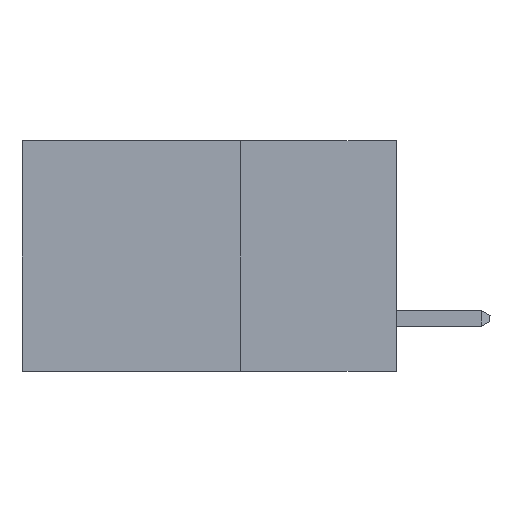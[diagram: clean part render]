
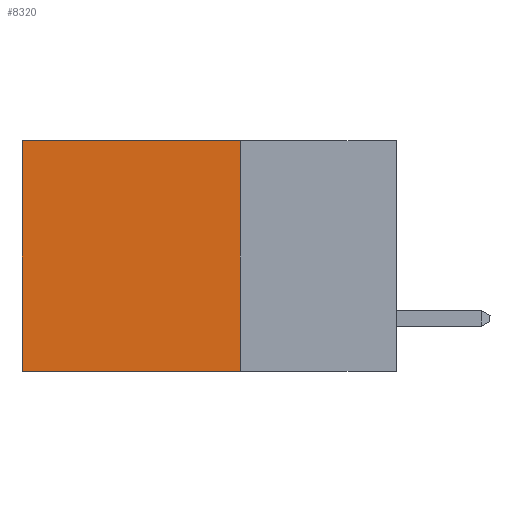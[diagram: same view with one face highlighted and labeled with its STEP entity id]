
A CAD part, left-side view. The second image highlights one B-rep face of the part: STEP entity #8320.
In plain terms, the highlighted planar face has unit normal (-1, 0, 0).
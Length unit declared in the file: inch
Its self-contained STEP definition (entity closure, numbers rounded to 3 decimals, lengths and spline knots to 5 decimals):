
#2865 = ORIENTED_EDGE ( 'NONE', *, *, #7196, .T. ) ;
#3158 = CARTESIAN_POINT ( 'NONE',  ( 0.2615, 0.25, -0.37 ) ) ;
#3187 = VERTEX_POINT ( 'NONE', #3698 ) ;
#3439 = EDGE_CURVE ( 'NONE', #10268, #3187, #15958, .T. ) ;
#3698 = CARTESIAN_POINT ( 'NONE',  ( 0.2615, 0.6, 0. ) ) ;
#4251 = VERTEX_POINT ( 'NONE', #8375 ) ;
#4569 = FACE_OUTER_BOUND ( 'NONE', #12228, .T. ) ;
#5017 = EDGE_CURVE ( 'NONE', #10268, #4251, #17143, .T. ) ;
#7196 = EDGE_CURVE ( 'NONE', #3187, #14662, #18807, .T. ) ;
#7210 = CARTESIAN_POINT ( 'NONE',  ( 0.2615, 0.6, -0.37 ) ) ;
#8123 = CARTESIAN_POINT ( 'NONE',  ( 0.2615, 0.6, -0.37 ) ) ;
#8320 = ADVANCED_FACE ( 'NONE', ( #4569 ), #22385, .F. ) ;
#8375 = CARTESIAN_POINT ( 'NONE',  ( 0.2615, 0.25, -0.37 ) ) ;
#9937 = DIRECTION ( 'NONE',  ( 1., 0., 0. ) ) ;
#10097 = CARTESIAN_POINT ( 'NONE',  ( 0.2615, 0.25, 0. ) ) ;
#10268 = VERTEX_POINT ( 'NONE', #22931 ) ;
#11072 = VECTOR ( 'NONE', #18693, 39.37008 ) ;
#11886 = LINE ( 'NONE', #3158, #18619 ) ;
#12228 = EDGE_LOOP ( 'NONE', ( #2865, #20661, #18060, #17676 ) ) ;
#12373 = VECTOR ( 'NONE', #20550, 39.37008 ) ;
#13511 = DIRECTION ( 'NONE',  ( 0., 0., -1. ) ) ;
#13871 = CARTESIAN_POINT ( 'NONE',  ( 0.2615, 0.25, -0.37 ) ) ;
#14662 = VERTEX_POINT ( 'NONE', #7210 ) ;
#15172 = DIRECTION ( 'NONE',  ( 0., 0., -1. ) ) ;
#15958 = LINE ( 'NONE', #10097, #12373 ) ;
#16049 = VECTOR ( 'NONE', #15172, 39.37008 ) ;
#17143 = LINE ( 'NONE', #13871, #16049 ) ;
#17676 = ORIENTED_EDGE ( 'NONE', *, *, #3439, .T. ) ;
#18060 = ORIENTED_EDGE ( 'NONE', *, *, #5017, .F. ) ;
#18619 = VECTOR ( 'NONE', #20616, 39.37008 ) ;
#18693 = DIRECTION ( 'NONE',  ( 0., 0., -1. ) ) ;
#18807 = LINE ( 'NONE', #8123, #11072 ) ;
#20550 = DIRECTION ( 'NONE',  ( 0., 1., 0. ) ) ;
#20616 = DIRECTION ( 'NONE',  ( 0., 1., 0. ) ) ;
#20661 = ORIENTED_EDGE ( 'NONE', *, *, #21427, .F. ) ;
#21427 = EDGE_CURVE ( 'NONE', #4251, #14662, #11886, .T. ) ;
#22311 = AXIS2_PLACEMENT_3D ( 'NONE', #22619, #9937, #13511 ) ;
#22385 = PLANE ( 'NONE',  #22311 ) ;
#22619 = CARTESIAN_POINT ( 'NONE',  ( 0.2615, 0.25, -0.37 ) ) ;
#22931 = CARTESIAN_POINT ( 'NONE',  ( 0.2615, 0.25, 0. ) ) ;
